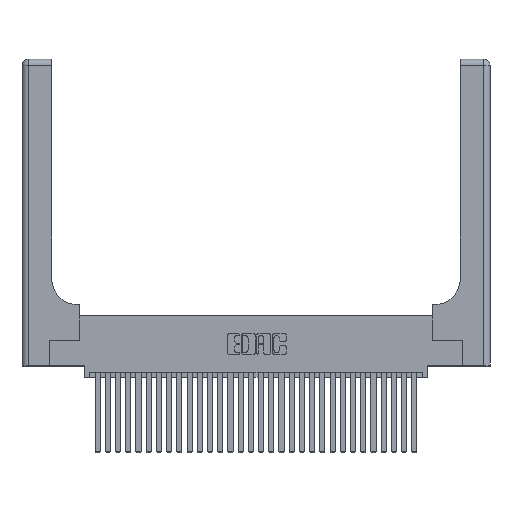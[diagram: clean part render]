
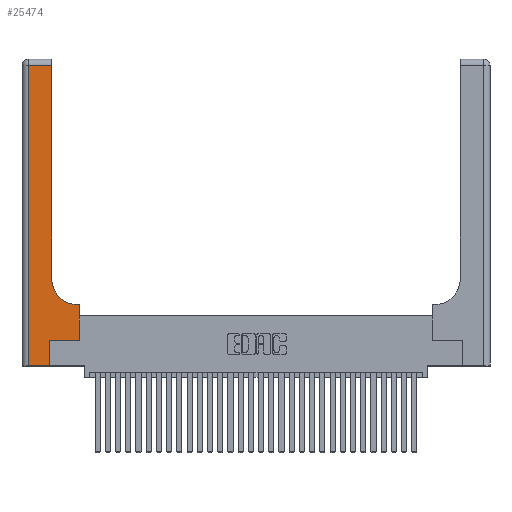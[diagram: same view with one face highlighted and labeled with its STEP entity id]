
A CAD part, top view. The second image highlights one B-rep face of the part: STEP entity #25474.
In plain terms, the highlighted planar face has unit normal (0, 0, 1).
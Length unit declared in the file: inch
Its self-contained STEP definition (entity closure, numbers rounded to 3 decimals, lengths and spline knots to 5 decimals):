
#158 = EDGE_CURVE ( 'NONE', #2675, #31605, #12864, .T. ) ;
#392 = VERTEX_POINT ( 'NONE', #10462 ) ;
#742 = CARTESIAN_POINT ( 'NONE',  ( 0.06, 2.94, 0.37 ) ) ;
#2121 = CARTESIAN_POINT ( 'NONE',  ( 0.5585, 0.25, 0.37 ) ) ;
#2398 = VERTEX_POINT ( 'NONE', #5267 ) ;
#2675 = VERTEX_POINT ( 'NONE', #23380 ) ;
#2832 = AXIS2_PLACEMENT_3D ( 'NONE', #17643, #17614, #17329 ) ;
#3052 = DIRECTION ( 'NONE',  ( -1., 0., 0. ) ) ;
#3101 = LINE ( 'NONE', #11352, #8863 ) ;
#4496 = ORIENTED_EDGE ( 'NONE', *, *, #23177, .T. ) ;
#5260 = VECTOR ( 'NONE', #29582, 39.37008 ) ;
#5267 = CARTESIAN_POINT ( 'NONE',  ( 0.06, 0., 0.37 ) ) ;
#5766 = CARTESIAN_POINT ( 'NONE',  ( 0.2915, 3., 0.37 ) ) ;
#6100 = EDGE_CURVE ( 'NONE', #26114, #392, #22242, .T. ) ;
#6150 = EDGE_CURVE ( 'NONE', #19250, #26114, #7696, .T. ) ;
#6679 = EDGE_CURVE ( 'NONE', #31605, #17003, #31215, .T. ) ;
#7696 = LINE ( 'NONE', #17260, #26345 ) ;
#8070 = CARTESIAN_POINT ( 'NONE',  ( 0.2915, 0.85, 0.37 ) ) ;
#8656 = LINE ( 'NONE', #10158, #20127 ) ;
#8846 = DIRECTION ( 'NONE',  ( 1., 0., 0. ) ) ;
#8863 = VECTOR ( 'NONE', #8846, 39.37008 ) ;
#9489 = DIRECTION ( 'NONE',  ( -1., 0., 0. ) ) ;
#10158 = CARTESIAN_POINT ( 'NONE',  ( 0.269, 0., 0.37 ) ) ;
#10462 = CARTESIAN_POINT ( 'NONE',  ( 0.5585, 0.6, 0.37 ) ) ;
#11348 = DIRECTION ( 'NONE',  ( -1., 0., 0. ) ) ;
#11352 = CARTESIAN_POINT ( 'NONE',  ( 0., 0., 0.37 ) ) ;
#11686 = VECTOR ( 'NONE', #11348, 39.37008 ) ;
#11694 = VERTEX_POINT ( 'NONE', #742 ) ;
#12076 = CARTESIAN_POINT ( 'NONE',  ( 0.269, 0., 0.37 ) ) ;
#12156 = ORIENTED_EDGE ( 'NONE', *, *, #6679, .T. ) ;
#12733 = CARTESIAN_POINT ( 'NONE',  ( 0.2915, 0.6, 0.37 ) ) ;
#12864 = CIRCLE ( 'NONE', #2832, 0.25 ) ;
#12927 = ORIENTED_EDGE ( 'NONE', *, *, #27738, .T. ) ;
#13327 = ORIENTED_EDGE ( 'NONE', *, *, #18575, .T. ) ;
#13622 = AXIS2_PLACEMENT_3D ( 'NONE', #21665, #24082, #9489 ) ;
#13664 = ORIENTED_EDGE ( 'NONE', *, *, #17686, .T. ) ;
#14119 = ORIENTED_EDGE ( 'NONE', *, *, #158, .T. ) ;
#14182 = PLANE ( 'NONE',  #13622 ) ;
#14454 = VERTEX_POINT ( 'NONE', #12076 ) ;
#14590 = CARTESIAN_POINT ( 'NONE',  ( 0.5585, 0.25, 0.37 ) ) ;
#14755 = FACE_OUTER_BOUND ( 'NONE', #29334, .T. ) ;
#15997 = ORIENTED_EDGE ( 'NONE', *, *, #23728, .T. ) ;
#17003 = VERTEX_POINT ( 'NONE', #18724 ) ;
#17260 = CARTESIAN_POINT ( 'NONE',  ( 0.269, 0.25, 0.37 ) ) ;
#17329 = DIRECTION ( 'NONE',  ( 1., 0., 0. ) ) ;
#17362 = LINE ( 'NONE', #12733, #29433 ) ;
#17614 = DIRECTION ( 'NONE',  ( 0., 0., -1. ) ) ;
#17643 = CARTESIAN_POINT ( 'NONE',  ( 0.5415, 0.85, 0.37 ) ) ;
#17686 = EDGE_CURVE ( 'NONE', #17003, #11694, #18932, .T. ) ;
#18248 = CARTESIAN_POINT ( 'NONE',  ( 0.269, 0.25, 0.37 ) ) ;
#18398 = VECTOR ( 'NONE', #27661, 39.37008 ) ;
#18575 = EDGE_CURVE ( 'NONE', #392, #2675, #17362, .T. ) ;
#18724 = CARTESIAN_POINT ( 'NONE',  ( 0.2915, 2.94, 0.37 ) ) ;
#18932 = LINE ( 'NONE', #28263, #11686 ) ;
#19250 = VERTEX_POINT ( 'NONE', #18248 ) ;
#19712 = DIRECTION ( 'NONE',  ( 1., 0., 0. ) ) ;
#20127 = VECTOR ( 'NONE', #21897, 39.37008 ) ;
#21472 = VECTOR ( 'NONE', #24388, 39.37008 ) ;
#21665 = CARTESIAN_POINT ( 'NONE',  ( 0., 3., 0.37 ) ) ;
#21897 = DIRECTION ( 'NONE',  ( 0., 1., 0. ) ) ;
#22242 = LINE ( 'NONE', #14590, #21472 ) ;
#23177 = EDGE_CURVE ( 'NONE', #11694, #2398, #24712, .T. ) ;
#23380 = CARTESIAN_POINT ( 'NONE',  ( 0.5415, 0.6, 0.37 ) ) ;
#23728 = EDGE_CURVE ( 'NONE', #14454, #19250, #8656, .T. ) ;
#24082 = DIRECTION ( 'NONE',  ( 0., 0., -1. ) ) ;
#24388 = DIRECTION ( 'NONE',  ( 0., 1., 0. ) ) ;
#24712 = LINE ( 'NONE', #27153, #5260 ) ;
#24761 = ORIENTED_EDGE ( 'NONE', *, *, #6100, .T. ) ;
#25474 = ADVANCED_FACE ( 'NONE', ( #14755 ), #14182, .F. ) ;
#26114 = VERTEX_POINT ( 'NONE', #2121 ) ;
#26345 = VECTOR ( 'NONE', #19712, 39.37008 ) ;
#27153 = CARTESIAN_POINT ( 'NONE',  ( 0.06, 3., 0.37 ) ) ;
#27661 = DIRECTION ( 'NONE',  ( 0., 1., 0. ) ) ;
#27738 = EDGE_CURVE ( 'NONE', #2398, #14454, #3101, .T. ) ;
#28263 = CARTESIAN_POINT ( 'NONE',  ( 0., 2.94, 0.37 ) ) ;
#29334 = EDGE_LOOP ( 'NONE', ( #12156, #13664, #4496, #12927, #15997, #29623, #24761, #13327, #14119 ) ) ;
#29433 = VECTOR ( 'NONE', #3052, 39.37008 ) ;
#29582 = DIRECTION ( 'NONE',  ( 0., -1., 0. ) ) ;
#29623 = ORIENTED_EDGE ( 'NONE', *, *, #6150, .T. ) ;
#31215 = LINE ( 'NONE', #5766, #18398 ) ;
#31605 = VERTEX_POINT ( 'NONE', #8070 ) ;
